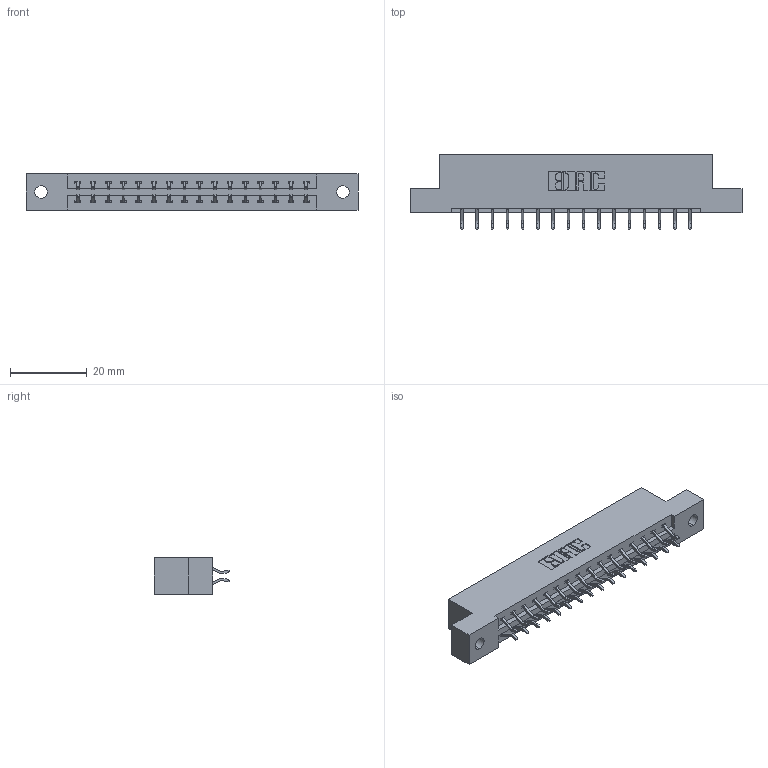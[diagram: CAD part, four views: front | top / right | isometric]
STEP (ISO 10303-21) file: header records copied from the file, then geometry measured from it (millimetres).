
FILE_DESCRIPTION (( 'STEP AP203' ), '1' );
FILE_NAME ('337-032-556-202.STEP', '2018-08-07T06:58:08', ( '' ), ( '' ), 'SwSTEP 2.0', 'SolidWorks 2016', '' );
FILE_SCHEMA (( 'CONFIG_CONTROL_DESIGN' ));
Length unit declared in the file: inch
Products named in the file (3): 337 Part_Flush Mounting Lugs - 0.128 Dia; 345-292-001_556 Tail; 337-032-556-202
Assembly tree (33 placements, depth 2):
  337-032-556-202
    337 Part_Flush Mounting Lugs - 0.128 Dia
    345-292-001_556 Tail  x32
Bounding box: 86.41 x 19.57 x 9.4 mm (x, y, z)
Volume: 8722.6 mm3; surface area: 9301.9 mm2
Topology: 33 solids, 33 shells, 2034 faces, 6039 edges, 3982 vertices
Faces by surface type: plane 1414, cylinder 620
Entity records: 15991 total; most frequent: CARTESIAN_POINT 2730, ORIENTED_EDGE 2654, DIRECTION 2359, EDGE_CURVE 1327, LINE 1191, VECTOR 1191, VERTEX_POINT 882, AXIS2_PLACEMENT_3D 584
